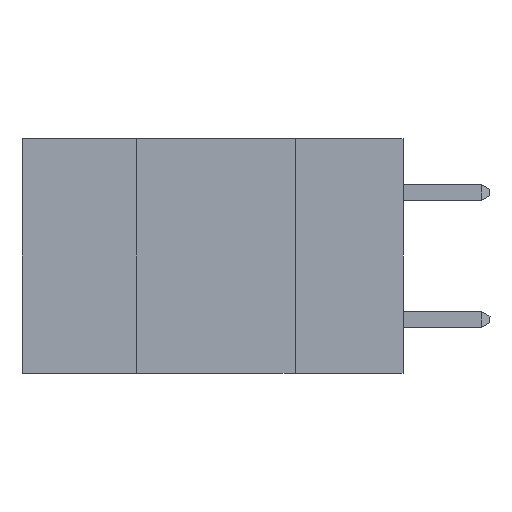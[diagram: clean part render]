
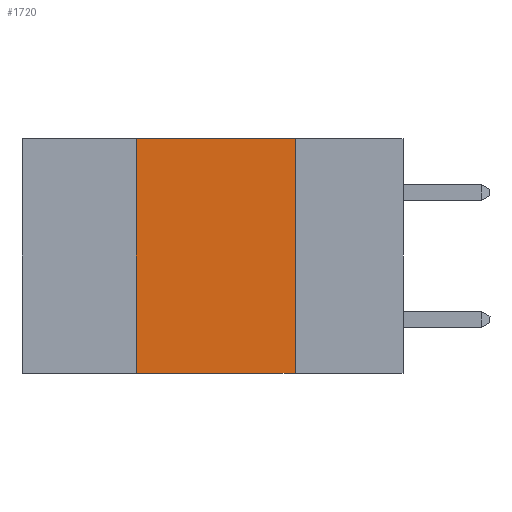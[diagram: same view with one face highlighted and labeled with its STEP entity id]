
A CAD part, left-side view. The second image highlights one B-rep face of the part: STEP entity #1720.
In plain terms, the highlighted planar face has unit normal (-1, 0, 0).
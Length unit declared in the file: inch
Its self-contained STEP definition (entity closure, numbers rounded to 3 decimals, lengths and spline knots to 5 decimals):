
#13 = ORIENTED_EDGE ( 'NONE', *, *, #6806, .T. ) ;
#76 = CARTESIAN_POINT ( 'NONE',  ( 0., 0.6, 0. ) ) ;
#121 = FACE_OUTER_BOUND ( 'NONE', #670, .T. ) ;
#670 = EDGE_LOOP ( 'NONE', ( #3789, #3395, #6173, #13 ) ) ;
#698 = LINE ( 'NONE', #8705, #8541 ) ;
#932 = CARTESIAN_POINT ( 'NONE',  ( 0., 0.42, -0.37 ) ) ;
#1481 = EDGE_CURVE ( 'NONE', #2822, #7509, #4060, .T. ) ;
#1482 = LINE ( 'NONE', #6180, #4597 ) ;
#1720 = ADVANCED_FACE ( 'NONE', ( #121 ), #8722, .F. ) ;
#2128 = DIRECTION ( 'NONE',  ( 0., -1., 0. ) ) ;
#2822 = VERTEX_POINT ( 'NONE', #932 ) ;
#3121 = CARTESIAN_POINT ( 'NONE',  ( 0., 0.17, 0. ) ) ;
#3395 = ORIENTED_EDGE ( 'NONE', *, *, #5020, .F. ) ;
#3789 = ORIENTED_EDGE ( 'NONE', *, *, #5893, .F. ) ;
#3968 = DIRECTION ( 'NONE',  ( 0., 0., 1. ) ) ;
#3979 = CARTESIAN_POINT ( 'NONE',  ( 0., 0.17, 0. ) ) ;
#4060 = LINE ( 'NONE', #7530, #4903 ) ;
#4088 = VERTEX_POINT ( 'NONE', #6604 ) ;
#4597 = VECTOR ( 'NONE', #4734, 39.37008 ) ;
#4609 = VERTEX_POINT ( 'NONE', #3979 ) ;
#4734 = DIRECTION ( 'NONE',  ( 0., -1., 0. ) ) ;
#4903 = VECTOR ( 'NONE', #3968, 39.37008 ) ;
#5020 = EDGE_CURVE ( 'NONE', #7509, #4609, #1482, .T. ) ;
#5250 = DIRECTION ( 'NONE',  ( 0., 0., -1. ) ) ;
#5893 = EDGE_CURVE ( 'NONE', #4609, #4088, #8313, .T. ) ;
#6173 = ORIENTED_EDGE ( 'NONE', *, *, #1481, .F. ) ;
#6180 = CARTESIAN_POINT ( 'NONE',  ( 0., 0.6, 0. ) ) ;
#6222 = CARTESIAN_POINT ( 'NONE',  ( 0., 0.42, 0. ) ) ;
#6604 = CARTESIAN_POINT ( 'NONE',  ( 0., 0.17, -0.37 ) ) ;
#6700 = DIRECTION ( 'NONE',  ( 1., 0., 0. ) ) ;
#6737 = VECTOR ( 'NONE', #8366, 39.37008 ) ;
#6806 = EDGE_CURVE ( 'NONE', #2822, #4088, #698, .T. ) ;
#7509 = VERTEX_POINT ( 'NONE', #6222 ) ;
#7530 = CARTESIAN_POINT ( 'NONE',  ( 0., 0.42, 0. ) ) ;
#7784 = AXIS2_PLACEMENT_3D ( 'NONE', #76, #6700, #5250 ) ;
#8313 = LINE ( 'NONE', #3121, #6737 ) ;
#8366 = DIRECTION ( 'NONE',  ( 0., 0., -1. ) ) ;
#8541 = VECTOR ( 'NONE', #2128, 39.37008 ) ;
#8705 = CARTESIAN_POINT ( 'NONE',  ( 0., 0.6, -0.37 ) ) ;
#8722 = PLANE ( 'NONE',  #7784 ) ;
